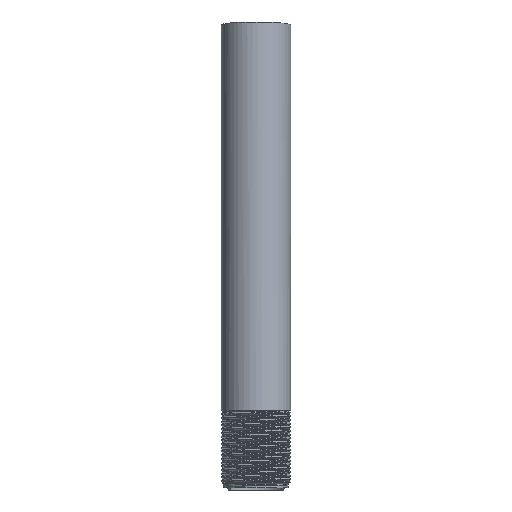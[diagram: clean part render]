
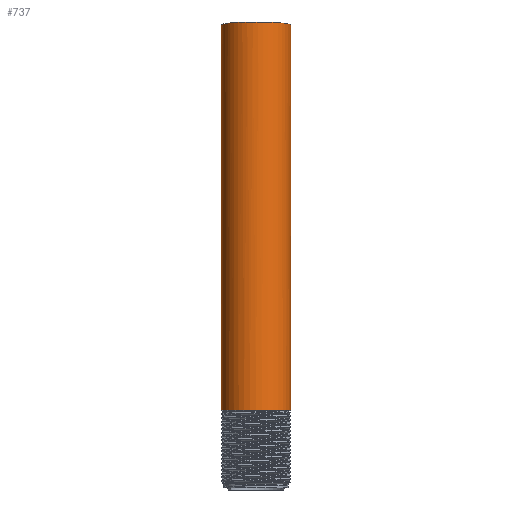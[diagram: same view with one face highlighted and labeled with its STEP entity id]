
A CAD part, front view. The second image highlights one B-rep face of the part: STEP entity #737.
In plain terms, the highlighted cylindrical face has radius 14.922 mm (diameter 29.845 mm), a partial arc.
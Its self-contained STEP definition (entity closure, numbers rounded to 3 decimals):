
#113 = VERTEX_POINT ( 'NONE', #6543 ) ;
#353 = ORIENTED_EDGE ( 'NONE', *, *, #8993, .T. ) ;
#651 = CARTESIAN_POINT ( 'NONE',  ( 14.922, 0., -1.306 ) ) ;
#737 = ADVANCED_FACE ( 'NONE', ( #5282 ), #15351, .T. ) ;
#1441 = VECTOR ( 'NONE', #12908, 1000. ) ;
#2041 = CARTESIAN_POINT ( 'NONE',  ( 0., 0., -165.848 ) ) ;
#2084 = EDGE_CURVE ( 'NONE', #113, #12947, #5418, .T. ) ;
#2498 = ORIENTED_EDGE ( 'NONE', *, *, #10115, .T. ) ;
#3078 = CARTESIAN_POINT ( 'NONE',  ( 0., 0., 0. ) ) ;
#3192 = CARTESIAN_POINT ( 'NONE',  ( -14.922, 0., -1.306 ) ) ;
#3319 = DIRECTION ( 'NONE',  ( 1., 0., 0. ) ) ;
#3769 = CARTESIAN_POINT ( 'NONE',  ( 14.922, 0., 0. ) ) ;
#4429 = DIRECTION ( 'NONE',  ( 1., 0., 0. ) ) ;
#4482 = CARTESIAN_POINT ( 'NONE',  ( -14.922, 0., -165.848 ) ) ;
#4691 = LINE ( 'NONE', #6987, #5079 ) ;
#5079 = VECTOR ( 'NONE', #8299, 1000. ) ;
#5282 = FACE_OUTER_BOUND ( 'NONE', #11516, .T. ) ;
#5418 =( BOUNDED_CURVE ( )  B_SPLINE_CURVE ( 3, ( #651, #10937, #10987, #3192 ),
 .UNSPECIFIED., .F., .F. ) 
 B_SPLINE_CURVE_WITH_KNOTS ( ( 4, 4 ),
 ( 4.712, 7.854 ),
 .UNSPECIFIED. ) 
 CURVE ( )  GEOMETRIC_REPRESENTATION_ITEM ( )  RATIONAL_B_SPLINE_CURVE ( ( 1., 0.333, 0.333, 1. ) ) 
 REPRESENTATION_ITEM ( '' )  );
#6543 = CARTESIAN_POINT ( 'NONE',  ( 14.922, 0., -1.306 ) ) ;
#6987 = CARTESIAN_POINT ( 'NONE',  ( -14.922, 0., 0. ) ) ;
#8299 = DIRECTION ( 'NONE',  ( 0., 0., 1. ) ) ;
#8434 = AXIS2_PLACEMENT_3D ( 'NONE', #2041, #11101, #3319 ) ;
#8626 = CARTESIAN_POINT ( 'NONE',  ( 14.922, 0., -165.848 ) ) ;
#8993 = EDGE_CURVE ( 'NONE', #10856, #15964, #9743, .T. ) ;
#9281 = ORIENTED_EDGE ( 'NONE', *, *, #2084, .T. ) ;
#9586 = AXIS2_PLACEMENT_3D ( 'NONE', #3078, #9765, #4429 ) ;
#9743 = CIRCLE ( 'NONE', #8434, 14.922 ) ;
#9765 = DIRECTION ( 'NONE',  ( 0., 0., 1. ) ) ;
#10115 = EDGE_CURVE ( 'NONE', #15964, #113, #14443, .T. ) ;
#10856 = VERTEX_POINT ( 'NONE', #4482 ) ;
#10891 = ORIENTED_EDGE ( 'NONE', *, *, #13948, .F. ) ;
#10937 = CARTESIAN_POINT ( 'NONE',  ( 14.923, -29.845, 1.306 ) ) ;
#10987 = CARTESIAN_POINT ( 'NONE',  ( -14.923, -29.845, 1.306 ) ) ;
#11101 = DIRECTION ( 'NONE',  ( 0., 0., 1. ) ) ;
#11516 = EDGE_LOOP ( 'NONE', ( #10891, #353, #2498, #9281 ) ) ;
#12675 = CARTESIAN_POINT ( 'NONE',  ( -14.922, 0., -1.306 ) ) ;
#12908 = DIRECTION ( 'NONE',  ( 0., 0., 1. ) ) ;
#12947 = VERTEX_POINT ( 'NONE', #12675 ) ;
#13948 = EDGE_CURVE ( 'NONE', #10856, #12947, #4691, .T. ) ;
#14443 = LINE ( 'NONE', #3769, #1441 ) ;
#15351 = CYLINDRICAL_SURFACE ( 'NONE', #9586, 14.922 ) ;
#15964 = VERTEX_POINT ( 'NONE', #8626 ) ;
